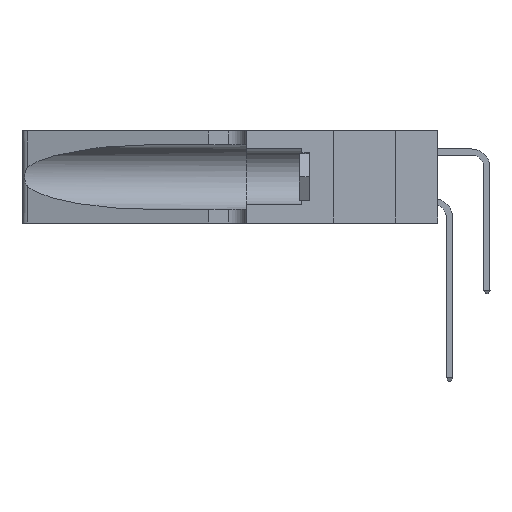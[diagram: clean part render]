
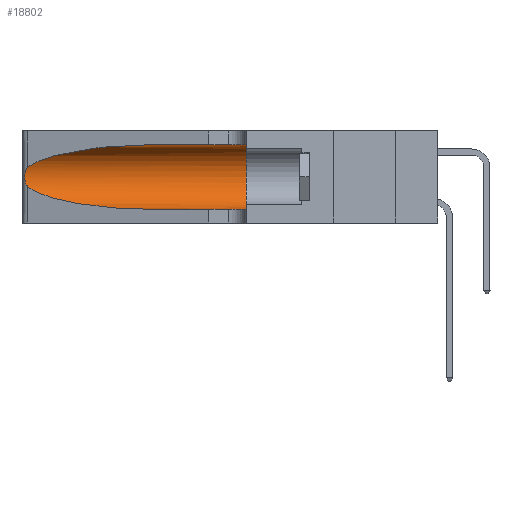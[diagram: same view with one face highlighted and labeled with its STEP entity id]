
A CAD part, left-side view. The second image highlights one B-rep face of the part: STEP entity #18802.
In plain terms, the highlighted cylindrical face has radius 3.308 mm (diameter 6.617 mm), a partial arc.
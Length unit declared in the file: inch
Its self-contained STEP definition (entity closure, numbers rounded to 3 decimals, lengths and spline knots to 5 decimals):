
#544 = CARTESIAN_POINT ( 'NONE',  ( 0.25555, 1.22994, 0.2215 ) ) ;
#563 = CARTESIAN_POINT ( 'NONE',  ( 0.2373, 1.15595, 0.08982 ) ) ;
#627 = CARTESIAN_POINT ( 'NONE',  ( 0.25555, 1.22993, 0.14849 ) ) ;
#953 = CARTESIAN_POINT ( 'NONE',  ( 0.1305, 1.61858, 0.185 ) ) ;
#1042 =( BOUNDED_CURVE ( )  B_SPLINE_CURVE ( 3, ( #10675, #8983, #14176, #3685 ),
 .UNSPECIFIED., .F., .F. ) 
 B_SPLINE_CURVE_WITH_KNOTS ( ( 4, 4 ),
 ( 1.5708, 2.84003 ),
 .UNSPECIFIED. ) 
 CURVE ( )  GEOMETRIC_REPRESENTATION_ITEM ( )  RATIONAL_B_SPLINE_CURVE ( ( 1., 0.87, 0.87, 1. ) ) 
 REPRESENTATION_ITEM ( '' )  );
#1347 = VERTEX_POINT ( 'NONE', #10977 ) ;
#1587 = AXIS2_PLACEMENT_3D ( 'NONE', #15991, #5658, #17676 ) ;
#3124 = DIRECTION ( 'NONE',  ( 0., -1., 0. ) ) ;
#3618 = DIRECTION ( 'NONE',  ( 0., -1., 0. ) ) ;
#3685 = CARTESIAN_POINT ( 'NONE',  ( 0.25487, 1.22718, 0.22369 ) ) ;
#4375 = CARTESIAN_POINT ( 'NONE',  ( 0.25787, 1.23484, 0.2124 ) ) ;
#5048 = VERTEX_POINT ( 'NONE', #22539 ) ;
#5658 = DIRECTION ( 'NONE',  ( 0., 1., 0. ) ) ;
#6165 = CARTESIAN_POINT ( 'NONE',  ( 0.26018, 1.23835, 0.19895 ) ) ;
#6174 = VERTEX_POINT ( 'NONE', #20107 ) ;
#6182 = CARTESIAN_POINT ( 'NONE',  ( 0.18966, 0.96281, 0.05475 ) ) ;
#6425 = EDGE_LOOP ( 'NONE', ( #22266, #7390, #18768, #11715, #8599, #9286 ) ) ;
#6475 = VECTOR ( 'NONE', #3618, 39.37008 ) ;
#6714 = EDGE_CURVE ( 'NONE', #9083, #6174, #7880, .T. ) ;
#6854 = VECTOR ( 'NONE', #3124, 39.37008 ) ;
#7342 =( BOUNDED_CURVE ( )  B_SPLINE_CURVE ( 3, ( #21497, #563, #6182, #18191 ),
 .UNSPECIFIED., .F., .F. ) 
 B_SPLINE_CURVE_WITH_KNOTS ( ( 4, 4 ),
 ( 3.44316, 4.71239 ),
 .UNSPECIFIED. ) 
 CURVE ( )  GEOMETRIC_REPRESENTATION_ITEM ( )  RATIONAL_B_SPLINE_CURVE ( ( 1., 0.87, 0.87, 1. ) ) 
 REPRESENTATION_ITEM ( '' )  );
#7390 = ORIENTED_EDGE ( 'NONE', *, *, #6714, .T. ) ;
#7839 = EDGE_CURVE ( 'NONE', #1347, #20942, #9051, .T. ) ;
#7880 = B_SPLINE_CURVE_WITH_KNOTS ( 'NONE', 3,
 ( #21485, #544, #14782, #4375, #16494, #6165, #18177, #7935, #19866, #9708, #21551, #11454, #627, #13164 ),
 .UNSPECIFIED., .F., .F.,
 ( 4, 2, 2, 2, 2, 2, 4 ),
 ( 0., 0.00027, 0.00053, 0.00107, 0.0016, 0.00187, 0.00214 ),
 .UNSPECIFIED. ) ;
#7935 = CARTESIAN_POINT ( 'NONE',  ( 0.26075, 1.23896, 0.178 ) ) ;
#8599 = ORIENTED_EDGE ( 'NONE', *, *, #7839, .F. ) ;
#8983 = CARTESIAN_POINT ( 'NONE',  ( 0.18966, 0.96281, 0.31525 ) ) ;
#9051 = CIRCLE ( 'NONE', #1587, 0.13025 ) ;
#9083 = VERTEX_POINT ( 'NONE', #16958 ) ;
#9157 = FACE_OUTER_BOUND ( 'NONE', #6425, .T. ) ;
#9286 = ORIENTED_EDGE ( 'NONE', *, *, #18043, .F. ) ;
#9584 = EDGE_CURVE ( 'NONE', #6174, #5048, #7342, .T. ) ;
#9708 = CARTESIAN_POINT ( 'NONE',  ( 0.25856, 1.23593, 0.16098 ) ) ;
#10675 = CARTESIAN_POINT ( 'NONE',  ( 0.1305, 0.72297, 0.31525 ) ) ;
#10977 = CARTESIAN_POINT ( 'NONE',  ( 0.1305, 0.35, 0.31525 ) ) ;
#11454 = CARTESIAN_POINT ( 'NONE',  ( 0.25639, 1.23186, 0.15144 ) ) ;
#11546 = VERTEX_POINT ( 'NONE', #16654 ) ;
#11654 = AXIS2_PLACEMENT_3D ( 'NONE', #953, #14303, #19396 ) ;
#11715 = ORIENTED_EDGE ( 'NONE', *, *, #14951, .T. ) ;
#12405 = CARTESIAN_POINT ( 'NONE',  ( 0.1305, 1.61858, 0.31525 ) ) ;
#13164 = CARTESIAN_POINT ( 'NONE',  ( 0.25487, 1.22718, 0.14631 ) ) ;
#13224 = CYLINDRICAL_SURFACE ( 'NONE', #11654, 0.13025 ) ;
#14176 = CARTESIAN_POINT ( 'NONE',  ( 0.2373, 1.15595, 0.28018 ) ) ;
#14303 = DIRECTION ( 'NONE',  ( 0., -1., 0. ) ) ;
#14707 = CARTESIAN_POINT ( 'NONE',  ( 0.1305, 0.35, 0.05475 ) ) ;
#14782 = CARTESIAN_POINT ( 'NONE',  ( 0.25639, 1.23184, 0.21858 ) ) ;
#14951 = EDGE_CURVE ( 'NONE', #5048, #20942, #20496, .T. ) ;
#15991 = CARTESIAN_POINT ( 'NONE',  ( 0.1305, 0.35, 0.185 ) ) ;
#16494 = CARTESIAN_POINT ( 'NONE',  ( 0.25854, 1.2359, 0.20912 ) ) ;
#16654 = CARTESIAN_POINT ( 'NONE',  ( 0.1305, 0.72297, 0.31525 ) ) ;
#16958 = CARTESIAN_POINT ( 'NONE',  ( 0.25487, 1.22718, 0.22369 ) ) ;
#17047 = CARTESIAN_POINT ( 'NONE',  ( 0.1305, 1.61858, 0.05475 ) ) ;
#17676 = DIRECTION ( 'NONE',  ( 0., 0., 1. ) ) ;
#18043 = EDGE_CURVE ( 'NONE', #11546, #1347, #19578, .T. ) ;
#18177 = CARTESIAN_POINT ( 'NONE',  ( 0.26075, 1.23896, 0.19203 ) ) ;
#18191 = CARTESIAN_POINT ( 'NONE',  ( 0.1305, 0.72297, 0.05475 ) ) ;
#18768 = ORIENTED_EDGE ( 'NONE', *, *, #9584, .T. ) ;
#18802 = ADVANCED_FACE ( 'NONE', ( #9157 ), #13224, .F. ) ;
#19396 = DIRECTION ( 'NONE',  ( 0., 0., -1. ) ) ;
#19578 = LINE ( 'NONE', #12405, #6475 ) ;
#19866 = CARTESIAN_POINT ( 'NONE',  ( 0.26017, 1.23833, 0.17102 ) ) ;
#20107 = CARTESIAN_POINT ( 'NONE',  ( 0.25487, 1.22718, 0.14631 ) ) ;
#20496 = LINE ( 'NONE', #17047, #6854 ) ;
#20942 = VERTEX_POINT ( 'NONE', #14707 ) ;
#21360 = EDGE_CURVE ( 'NONE', #11546, #9083, #1042, .T. ) ;
#21485 = CARTESIAN_POINT ( 'NONE',  ( 0.25487, 1.22718, 0.22369 ) ) ;
#21497 = CARTESIAN_POINT ( 'NONE',  ( 0.25487, 1.22718, 0.14631 ) ) ;
#21551 = CARTESIAN_POINT ( 'NONE',  ( 0.25789, 1.23486, 0.15765 ) ) ;
#22266 = ORIENTED_EDGE ( 'NONE', *, *, #21360, .T. ) ;
#22539 = CARTESIAN_POINT ( 'NONE',  ( 0.1305, 0.72297, 0.05475 ) ) ;
